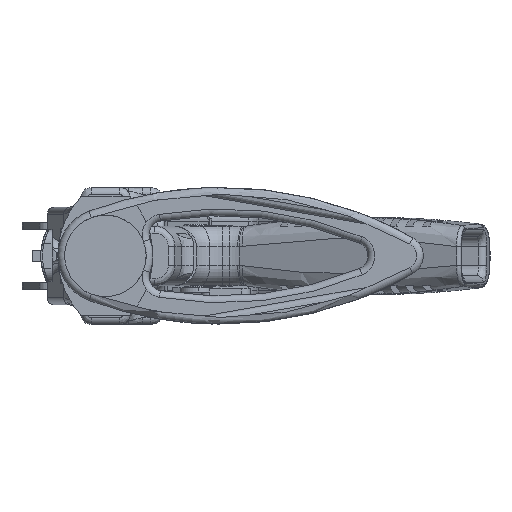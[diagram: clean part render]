
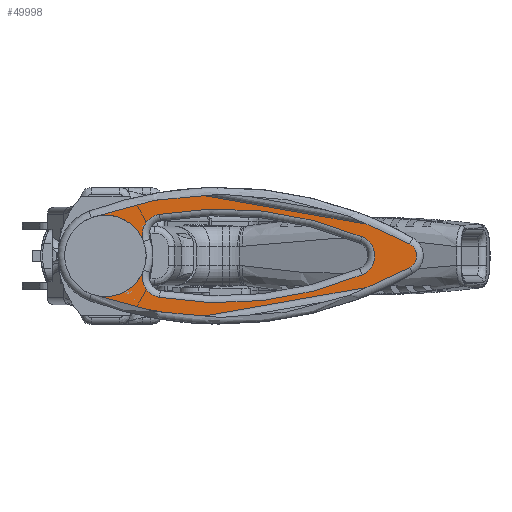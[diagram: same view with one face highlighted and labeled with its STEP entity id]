
A CAD part, left-side view. The second image highlights one B-rep face of the part: STEP entity #49998.
In plain terms, the highlighted planar face has unit normal (1, 0, 0).
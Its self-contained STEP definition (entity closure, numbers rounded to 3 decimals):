
#2456=PLANE('',#53993);
#15553=FACE_OUTER_BOUND('',#18555,.T.);
#18555=EDGE_LOOP('',(#46869,#46870,#46871,#46872,#46873,#46874,#46875,#46876,
#46877,#46878,#46879));
#20017=CIRCLE('',#53975,5.304);
#20019=CIRCLE('',#53978,0.3);
#20025=CIRCLE('',#53986,0.3);
#20028=CIRCLE('',#53990,5.304);
#20029=CIRCLE('',#53992,0.3);
#20030=CIRCLE('',#53994,0.595);
#20031=CIRCLE('',#53995,0.595);
#20032=CIRCLE('',#53996,5.517);
#20033=CIRCLE('',#53997,0.2);
#20034=CIRCLE('',#53998,5.517);
#20035=CIRCLE('',#53999,0.595);
#24757=VERTEX_POINT('',#146830);
#24758=VERTEX_POINT('',#146832);
#24760=VERTEX_POINT('',#146837);
#24762=VERTEX_POINT('',#146844);
#24763=VERTEX_POINT('',#146848);
#24764=VERTEX_POINT('',#146853);
#24765=VERTEX_POINT('',#146859);
#24766=VERTEX_POINT('',#146861);
#24767=VERTEX_POINT('',#146863);
#24768=VERTEX_POINT('',#146865);
#24769=VERTEX_POINT('',#146867);
#32137=EDGE_CURVE('',#24758,#24757,#20017,.T.);
#32139=EDGE_CURVE('',#24760,#24758,#20019,.T.);
#32145=EDGE_CURVE('',#24763,#24762,#20025,.T.);
#32148=EDGE_CURVE('',#24764,#24763,#20028,.T.);
#32149=EDGE_CURVE('',#24757,#24764,#20029,.T.);
#32150=EDGE_CURVE('',#24760,#24765,#20030,.T.);
#32151=EDGE_CURVE('',#24765,#24766,#20031,.T.);
#32152=EDGE_CURVE('',#24767,#24766,#20032,.T.);
#32153=EDGE_CURVE('',#24768,#24767,#20033,.T.);
#32154=EDGE_CURVE('',#24769,#24768,#20034,.T.);
#32155=EDGE_CURVE('',#24769,#24762,#20035,.T.);
#46869=ORIENTED_EDGE('',*,*,#32145,.F.);
#46870=ORIENTED_EDGE('',*,*,#32148,.F.);
#46871=ORIENTED_EDGE('',*,*,#32149,.F.);
#46872=ORIENTED_EDGE('',*,*,#32137,.F.);
#46873=ORIENTED_EDGE('',*,*,#32139,.F.);
#46874=ORIENTED_EDGE('',*,*,#32150,.T.);
#46875=ORIENTED_EDGE('',*,*,#32151,.T.);
#46876=ORIENTED_EDGE('',*,*,#32152,.F.);
#46877=ORIENTED_EDGE('',*,*,#32153,.F.);
#46878=ORIENTED_EDGE('',*,*,#32154,.F.);
#46879=ORIENTED_EDGE('',*,*,#32155,.T.);
#49998=ADVANCED_FACE('',(#15553),#2456,.T.);
#53975=AXIS2_PLACEMENT_3D('',#146834,#65025,#65026);
#53978=AXIS2_PLACEMENT_3D('',#146839,#65031,#65032);
#53986=AXIS2_PLACEMENT_3D('',#146850,#65047,#65048);
#53990=AXIS2_PLACEMENT_3D('',#146855,#65055,#65056);
#53992=AXIS2_PLACEMENT_3D('',#146857,#65059,#65060);
#53993=AXIS2_PLACEMENT_3D('',#146858,#65061,#65062);
#53994=AXIS2_PLACEMENT_3D('',#146860,#65063,#65064);
#53995=AXIS2_PLACEMENT_3D('',#146862,#65065,#65066);
#53996=AXIS2_PLACEMENT_3D('',#146864,#65067,#65068);
#53997=AXIS2_PLACEMENT_3D('',#146866,#65069,#65070);
#53998=AXIS2_PLACEMENT_3D('',#146868,#65071,#65072);
#53999=AXIS2_PLACEMENT_3D('',#146869,#65073,#65074);
#65025=DIRECTION('center_axis',(1.,0.,0.));
#65026=DIRECTION('ref_axis',(0.,-0.11,0.994));
#65031=DIRECTION('center_axis',(1.,0.,0.));
#65032=DIRECTION('ref_axis',(0.,0.867,0.498));
#65047=DIRECTION('center_axis',(1.,0.,0.));
#65048=DIRECTION('ref_axis',(0.,0.867,-0.498));
#65055=DIRECTION('center_axis',(1.,0.,0.));
#65056=DIRECTION('ref_axis',(0.,-0.11,-0.994));
#65059=DIRECTION('center_axis',(1.,0.,0.));
#65060=DIRECTION('ref_axis',(0.,-1.,0.));
#65061=DIRECTION('center_axis',(1.,0.,0.));
#65062=DIRECTION('ref_axis',(0.,0.,-1.));
#65063=DIRECTION('center_axis',(-1.,0.,0.));
#65064=DIRECTION('ref_axis',(0.,0.,-1.));
#65065=DIRECTION('center_axis',(-1.,0.,0.));
#65066=DIRECTION('ref_axis',(0.,0.,-1.));
#65067=DIRECTION('center_axis',(-1.,0.,0.));
#65068=DIRECTION('ref_axis',(0.,-0.126,0.992));
#65069=DIRECTION('center_axis',(-1.,0.,0.));
#65070=DIRECTION('ref_axis',(0.,-1.,0.));
#65071=DIRECTION('center_axis',(-1.,0.,0.));
#65072=DIRECTION('ref_axis',(0.,-0.126,-0.992));
#65073=DIRECTION('center_axis',(-1.,0.,0.));
#65074=DIRECTION('ref_axis',(0.,0.,-1.));
#146830=CARTESIAN_POINT('',(0.975,-3.749,0.277));
#146832=CARTESIAN_POINT('',(0.975,-0.787,0.606));
#146834=CARTESIAN_POINT('Origin',(0.975,-1.706,-4.617));
#146837=CARTESIAN_POINT('',(0.975,-0.558,0.206));
#146839=CARTESIAN_POINT('Origin',(0.975,-0.839,0.311));
#146844=CARTESIAN_POINT('',(0.975,-0.558,-0.206));
#146848=CARTESIAN_POINT('',(0.975,-0.787,-0.606));
#146850=CARTESIAN_POINT('Origin',(0.975,-0.839,-0.311));
#146853=CARTESIAN_POINT('',(0.975,-3.749,-0.277));
#146855=CARTESIAN_POINT('Origin',(0.975,-1.706,4.617));
#146857=CARTESIAN_POINT('Origin',(0.975,-3.633,0.));
#146858=CARTESIAN_POINT('Origin',(0.975,-2.105,0.));
#146859=CARTESIAN_POINT('',(0.975,0.,0.595));
#146860=CARTESIAN_POINT('Origin',(0.975,0.,0.));
#146861=CARTESIAN_POINT('',(0.975,0.206,0.558));
#146862=CARTESIAN_POINT('Origin',(0.975,0.,0.));
#146863=CARTESIAN_POINT('',(0.975,-4.442,0.174));
#146864=CARTESIAN_POINT('Origin',(0.975,-1.706,-4.617));
#146865=CARTESIAN_POINT('',(0.975,-4.442,-0.174));
#146866=CARTESIAN_POINT('Origin',(0.975,-4.343,0.));
#146867=CARTESIAN_POINT('',(0.975,0.206,-0.558));
#146868=CARTESIAN_POINT('Origin',(0.975,-1.706,4.617));
#146869=CARTESIAN_POINT('Origin',(0.975,0.,0.));
